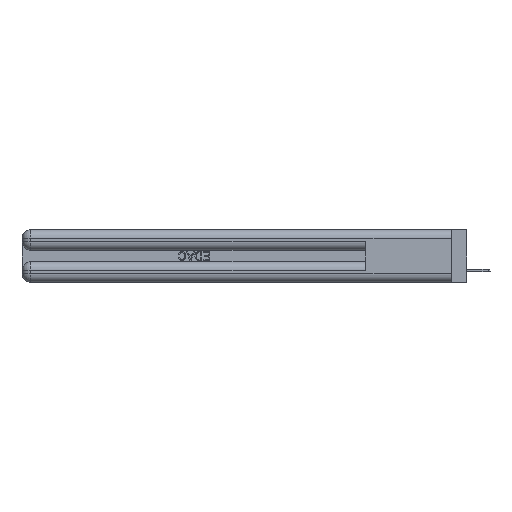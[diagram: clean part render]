
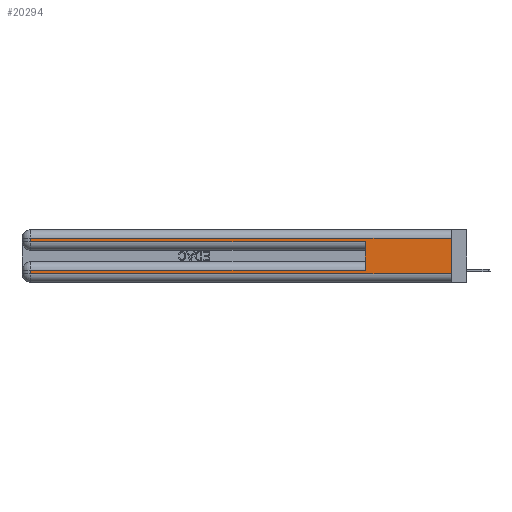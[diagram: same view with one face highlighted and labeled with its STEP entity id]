
A CAD part, left-side view. The second image highlights one B-rep face of the part: STEP entity #20294.
In plain terms, the highlighted planar face has unit normal (-1, 0, 0).
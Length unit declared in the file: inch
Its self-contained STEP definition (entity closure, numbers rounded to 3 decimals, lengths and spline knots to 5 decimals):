
#7 = LINE ( 'NONE', #3462, #16703 ) ;
#689 = VERTEX_POINT ( 'NONE', #16588 ) ;
#1350 = VERTEX_POINT ( 'NONE', #14868 ) ;
#1527 = CARTESIAN_POINT ( 'NONE',  ( 0., 2.94, 0.285 ) ) ;
#2428 = LINE ( 'NONE', #41022, #18461 ) ;
#2446 = LINE ( 'NONE', #46730, #23420 ) ;
#2677 = VECTOR ( 'NONE', #14148, 39.37008 ) ;
#3462 = CARTESIAN_POINT ( 'NONE',  ( 0., 2.94, 0.37 ) ) ;
#4256 = VERTEX_POINT ( 'NONE', #41709 ) ;
#4492 = ORIENTED_EDGE ( 'NONE', *, *, #37931, .F. ) ;
#5416 = EDGE_CURVE ( 'NONE', #44679, #1350, #2446, .T. ) ;
#6210 = CARTESIAN_POINT ( 'NONE',  ( 0., 0.6, 0.145 ) ) ;
#6525 = VERTEX_POINT ( 'NONE', #47356 ) ;
#7612 = VERTEX_POINT ( 'NONE', #21734 ) ;
#8914 = VECTOR ( 'NONE', #34189, 39.37008 ) ;
#10408 = LINE ( 'NONE', #45852, #40103 ) ;
#11489 = DIRECTION ( 'NONE',  ( 0., 0., -1. ) ) ;
#11556 = ORIENTED_EDGE ( 'NONE', *, *, #17023, .T. ) ;
#12966 = CARTESIAN_POINT ( 'NONE',  ( 0., 2.94, 0.085 ) ) ;
#14047 = CARTESIAN_POINT ( 'NONE',  ( 0., 0., 0.085 ) ) ;
#14148 = DIRECTION ( 'NONE',  ( 0., 0., 1. ) ) ;
#14868 = CARTESIAN_POINT ( 'NONE',  ( 0., 0., 0.06 ) ) ;
#15146 = EDGE_LOOP ( 'NONE', ( #45466, #28467, #26048, #11556, #4492, #41816, #30604, #36234 ) ) ;
#16588 = CARTESIAN_POINT ( 'NONE',  ( 0., 0.6, 0.085 ) ) ;
#16703 = VECTOR ( 'NONE', #19132, 39.37008 ) ;
#16985 = DIRECTION ( 'NONE',  ( 0., -1., 0. ) ) ;
#17023 = EDGE_CURVE ( 'NONE', #33275, #6525, #2428, .T. ) ;
#17564 = DIRECTION ( 'NONE',  ( 0., 1., 0. ) ) ;
#18107 = EDGE_CURVE ( 'NONE', #44679, #7612, #23859, .T. ) ;
#18461 = VECTOR ( 'NONE', #16985, 39.37008 ) ;
#18971 = DIRECTION ( 'NONE',  ( 0., 0., -1. ) ) ;
#19132 = DIRECTION ( 'NONE',  ( 0., 0., -1. ) ) ;
#20294 = ADVANCED_FACE ( 'NONE', ( #31565 ), #38723, .F. ) ;
#21734 = CARTESIAN_POINT ( 'NONE',  ( 0., 2.94, 0.31 ) ) ;
#22594 = CARTESIAN_POINT ( 'NONE',  ( 0., 2.94, 0.37 ) ) ;
#23420 = VECTOR ( 'NONE', #11489, 39.37008 ) ;
#23859 = LINE ( 'NONE', #41607, #29438 ) ;
#26048 = ORIENTED_EDGE ( 'NONE', *, *, #30132, .T. ) ;
#26881 = EDGE_CURVE ( 'NONE', #689, #45047, #49837, .T. ) ;
#27136 = AXIS2_PLACEMENT_3D ( 'NONE', #30549, #50422, #18971 ) ;
#28467 = ORIENTED_EDGE ( 'NONE', *, *, #18107, .T. ) ;
#29438 = VECTOR ( 'NONE', #17564, 39.37008 ) ;
#29973 = LINE ( 'NONE', #22594, #8914 ) ;
#30132 = EDGE_CURVE ( 'NONE', #7612, #33275, #7, .T. ) ;
#30549 = CARTESIAN_POINT ( 'NONE',  ( 0., 0., 0.37 ) ) ;
#30604 = ORIENTED_EDGE ( 'NONE', *, *, #37074, .T. ) ;
#31271 = VECTOR ( 'NONE', #49952, 39.37008 ) ;
#31565 = FACE_OUTER_BOUND ( 'NONE', #15146, .T. ) ;
#33275 = VERTEX_POINT ( 'NONE', #1527 ) ;
#33742 = CARTESIAN_POINT ( 'NONE',  ( 0., 0., 0.31 ) ) ;
#34101 = DIRECTION ( 'NONE',  ( 0., -1., 0. ) ) ;
#34189 = DIRECTION ( 'NONE',  ( 0., 0., -1. ) ) ;
#34850 = LINE ( 'NONE', #6210, #2677 ) ;
#36234 = ORIENTED_EDGE ( 'NONE', *, *, #49144, .T. ) ;
#37074 = EDGE_CURVE ( 'NONE', #45047, #4256, #29973, .T. ) ;
#37931 = EDGE_CURVE ( 'NONE', #689, #6525, #34850, .T. ) ;
#38723 = PLANE ( 'NONE',  #27136 ) ;
#40103 = VECTOR ( 'NONE', #34101, 39.37008 ) ;
#41022 = CARTESIAN_POINT ( 'NONE',  ( 0., 0., 0.285 ) ) ;
#41607 = CARTESIAN_POINT ( 'NONE',  ( 0., 0., 0.31 ) ) ;
#41709 = CARTESIAN_POINT ( 'NONE',  ( 0., 2.94, 0.06 ) ) ;
#41816 = ORIENTED_EDGE ( 'NONE', *, *, #26881, .T. ) ;
#44679 = VERTEX_POINT ( 'NONE', #33742 ) ;
#45047 = VERTEX_POINT ( 'NONE', #12966 ) ;
#45466 = ORIENTED_EDGE ( 'NONE', *, *, #5416, .F. ) ;
#45852 = CARTESIAN_POINT ( 'NONE',  ( 0., 0., 0.06 ) ) ;
#46730 = CARTESIAN_POINT ( 'NONE',  ( 0., 0., 0.37 ) ) ;
#47356 = CARTESIAN_POINT ( 'NONE',  ( 0., 0.6, 0.285 ) ) ;
#49144 = EDGE_CURVE ( 'NONE', #4256, #1350, #10408, .T. ) ;
#49837 = LINE ( 'NONE', #14047, #31271 ) ;
#49952 = DIRECTION ( 'NONE',  ( 0., 1., 0. ) ) ;
#50422 = DIRECTION ( 'NONE',  ( 1., 0., 0. ) ) ;
